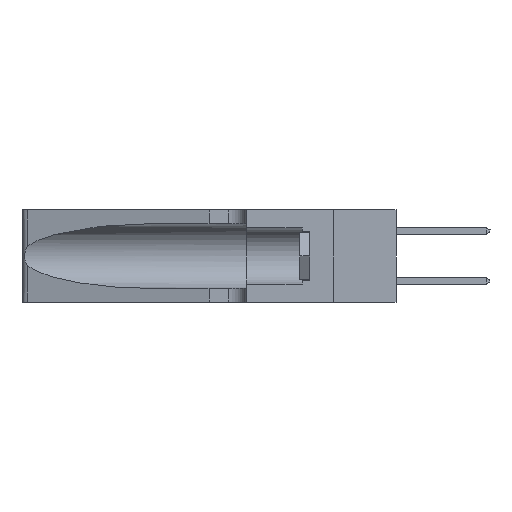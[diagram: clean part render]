
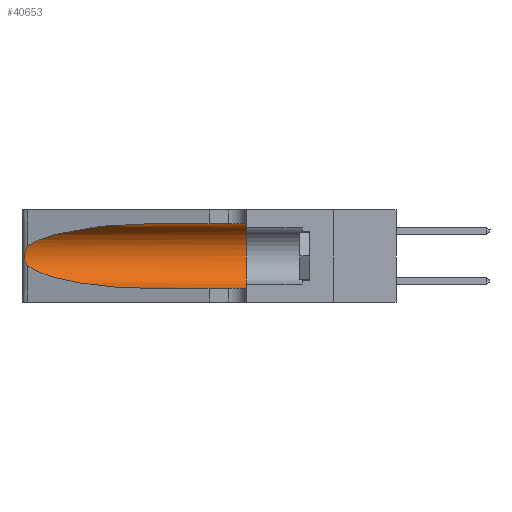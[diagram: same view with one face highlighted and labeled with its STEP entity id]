
A CAD part, left-side view. The second image highlights one B-rep face of the part: STEP entity #40653.
In plain terms, the highlighted cylindrical face has radius 3.308 mm (diameter 6.617 mm), a partial arc.
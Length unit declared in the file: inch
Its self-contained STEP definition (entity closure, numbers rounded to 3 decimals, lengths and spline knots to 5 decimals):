
#286 = DIRECTION ( 'NONE',  ( 0., 0., 1. ) ) ;
#1796 = CARTESIAN_POINT ( 'NONE',  ( 0.25787, 1.23484, 0.2124 ) ) ;
#2253 = ORIENTED_EDGE ( 'NONE', *, *, #13793, .F. ) ;
#3050 =( BOUNDED_CURVE ( )  B_SPLINE_CURVE ( 3, ( #19696, #16229, #5884, #30139 ),
 .UNSPECIFIED., .F., .T. ) 
 B_SPLINE_CURVE_WITH_KNOTS ( ( 4, 4 ),
 ( 3.44316, 4.71239 ),
 .UNSPECIFIED. ) 
 CURVE ( )  GEOMETRIC_REPRESENTATION_ITEM ( )  RATIONAL_B_SPLINE_CURVE ( ( 1., 0.87, 0.87, 1. ) ) 
 REPRESENTATION_ITEM ( '' )  );
#3281 = EDGE_CURVE ( 'NONE', #15753, #24183, #35313, .T. ) ;
#4783 = ORIENTED_EDGE ( 'NONE', *, *, #9770, .T. ) ;
#4801 = VERTEX_POINT ( 'NONE', #29005 ) ;
#5259 = CARTESIAN_POINT ( 'NONE',  ( 0.26018, 1.23835, 0.19895 ) ) ;
#5474 = CARTESIAN_POINT ( 'NONE',  ( 0.25487, 1.22718, 0.22369 ) ) ;
#5884 = CARTESIAN_POINT ( 'NONE',  ( 0.18966, 0.96281, 0.05475 ) ) ;
#8203 = ORIENTED_EDGE ( 'NONE', *, *, #8960, .T. ) ;
#8470 = DIRECTION ( 'NONE',  ( 0., -1., 0. ) ) ;
#8491 = VERTEX_POINT ( 'NONE', #29771 ) ;
#8501 = LINE ( 'NONE', #15479, #16653 ) ;
#8744 = CARTESIAN_POINT ( 'NONE',  ( 0.26075, 1.23896, 0.178 ) ) ;
#8960 = EDGE_CURVE ( 'NONE', #8491, #19997, #29274, .T. ) ;
#9373 = AXIS2_PLACEMENT_3D ( 'NONE', #25709, #29200, #18765 ) ;
#9770 = EDGE_CURVE ( 'NONE', #24183, #8491, #3050, .T. ) ;
#12256 = CARTESIAN_POINT ( 'NONE',  ( 0.25856, 1.23593, 0.16098 ) ) ;
#13555 = EDGE_LOOP ( 'NONE', ( #35148, #41933, #4783, #8203, #2253, #16869 ) ) ;
#13793 = EDGE_CURVE ( 'NONE', #4801, #19997, #22857, .T. ) ;
#15430 = EDGE_CURVE ( 'NONE', #27059, #15753, #23870, .T. ) ;
#15479 = CARTESIAN_POINT ( 'NONE',  ( 0.1305, 1.61858, 0.31525 ) ) ;
#15601 = CARTESIAN_POINT ( 'NONE',  ( 0.25639, 1.23184, 0.21858 ) ) ;
#15751 = CARTESIAN_POINT ( 'NONE',  ( 0.25639, 1.23186, 0.15144 ) ) ;
#15753 = VERTEX_POINT ( 'NONE', #17436 ) ;
#16229 = CARTESIAN_POINT ( 'NONE',  ( 0.2373, 1.15595, 0.08982 ) ) ;
#16653 = VECTOR ( 'NONE', #8470, 39.37008 ) ;
#16869 = ORIENTED_EDGE ( 'NONE', *, *, #37093, .F. ) ;
#17436 = CARTESIAN_POINT ( 'NONE',  ( 0.25487, 1.22718, 0.22369 ) ) ;
#18765 = DIRECTION ( 'NONE',  ( 0., 0., -1. ) ) ;
#18981 = VECTOR ( 'NONE', #21728, 39.37008 ) ;
#19208 = CARTESIAN_POINT ( 'NONE',  ( 0.25487, 1.22718, 0.14631 ) ) ;
#19696 = CARTESIAN_POINT ( 'NONE',  ( 0.25487, 1.22718, 0.14631 ) ) ;
#19997 = VERTEX_POINT ( 'NONE', #25529 ) ;
#21050 = DIRECTION ( 'NONE',  ( 0., 1., 0. ) ) ;
#21345 = CARTESIAN_POINT ( 'NONE',  ( 0.25487, 1.22718, 0.14631 ) ) ;
#21728 = DIRECTION ( 'NONE',  ( 0., -1., 0. ) ) ;
#22745 = CARTESIAN_POINT ( 'NONE',  ( 0.18966, 0.96281, 0.31525 ) ) ;
#22857 = CIRCLE ( 'NONE', #27629, 0.13025 ) ;
#23870 =( BOUNDED_CURVE ( )  B_SPLINE_CURVE ( 3, ( #43522, #22745, #26235, #5474 ),
 .UNSPECIFIED., .F., .F. ) 
 B_SPLINE_CURVE_WITH_KNOTS ( ( 4, 4 ),
 ( 1.5708, 2.84003 ),
 .UNSPECIFIED. ) 
 CURVE ( )  GEOMETRIC_REPRESENTATION_ITEM ( )  RATIONAL_B_SPLINE_CURVE ( ( 1., 0.87, 0.87, 1. ) ) 
 REPRESENTATION_ITEM ( '' )  );
#24183 = VERTEX_POINT ( 'NONE', #21345 ) ;
#25529 = CARTESIAN_POINT ( 'NONE',  ( 0.1305, 0.35, 0.05475 ) ) ;
#25709 = CARTESIAN_POINT ( 'NONE',  ( 0.1305, 1.61858, 0.185 ) ) ;
#26031 = CARTESIAN_POINT ( 'NONE',  ( 0.25854, 1.2359, 0.20912 ) ) ;
#26235 = CARTESIAN_POINT ( 'NONE',  ( 0.2373, 1.15595, 0.28018 ) ) ;
#27059 = VERTEX_POINT ( 'NONE', #32589 ) ;
#27629 = AXIS2_PLACEMENT_3D ( 'NONE', #41821, #21050, #286 ) ;
#29005 = CARTESIAN_POINT ( 'NONE',  ( 0.1305, 0.35, 0.31525 ) ) ;
#29200 = DIRECTION ( 'NONE',  ( 0., -1., 0. ) ) ;
#29274 = LINE ( 'NONE', #32037, #18981 ) ;
#29509 = CARTESIAN_POINT ( 'NONE',  ( 0.26075, 1.23896, 0.19203 ) ) ;
#29771 = CARTESIAN_POINT ( 'NONE',  ( 0.1305, 0.72297, 0.05475 ) ) ;
#30139 = CARTESIAN_POINT ( 'NONE',  ( 0.1305, 0.72297, 0.05475 ) ) ;
#32037 = CARTESIAN_POINT ( 'NONE',  ( 0.1305, 1.61858, 0.05475 ) ) ;
#32589 = CARTESIAN_POINT ( 'NONE',  ( 0.1305, 0.72297, 0.31525 ) ) ;
#33003 = CARTESIAN_POINT ( 'NONE',  ( 0.26017, 1.23833, 0.17102 ) ) ;
#35148 = ORIENTED_EDGE ( 'NONE', *, *, #15430, .T. ) ;
#35313 = B_SPLINE_CURVE_WITH_KNOTS ( 'NONE', 3,
 ( #43313, #36372, #15601, #1796, #26031, #5259, #29509, #8744, #33003, #12256, #36522, #15751, #39997, #19208 ),
 .UNSPECIFIED., .F., .F.,
 ( 4, 2, 2, 2, 2, 2, 4 ),
 ( 0., 0.00027, 0.00053, 0.00107, 0.0016, 0.00187, 0.00214 ),
 .UNSPECIFIED. ) ;
#36372 = CARTESIAN_POINT ( 'NONE',  ( 0.25555, 1.22994, 0.2215 ) ) ;
#36522 = CARTESIAN_POINT ( 'NONE',  ( 0.25789, 1.23486, 0.15765 ) ) ;
#37093 = EDGE_CURVE ( 'NONE', #27059, #4801, #8501, .T. ) ;
#39997 = CARTESIAN_POINT ( 'NONE',  ( 0.25555, 1.22993, 0.14849 ) ) ;
#40653 = ADVANCED_FACE ( 'NONE', ( #43967 ), #41794, .F. ) ;
#41794 = CYLINDRICAL_SURFACE ( 'NONE', #9373, 0.13025 ) ;
#41821 = CARTESIAN_POINT ( 'NONE',  ( 0.1305, 0.35, 0.185 ) ) ;
#41933 = ORIENTED_EDGE ( 'NONE', *, *, #3281, .T. ) ;
#43313 = CARTESIAN_POINT ( 'NONE',  ( 0.25487, 1.22718, 0.22369 ) ) ;
#43522 = CARTESIAN_POINT ( 'NONE',  ( 0.1305, 0.72297, 0.31525 ) ) ;
#43967 = FACE_OUTER_BOUND ( 'NONE', #13555, .T. ) ;
